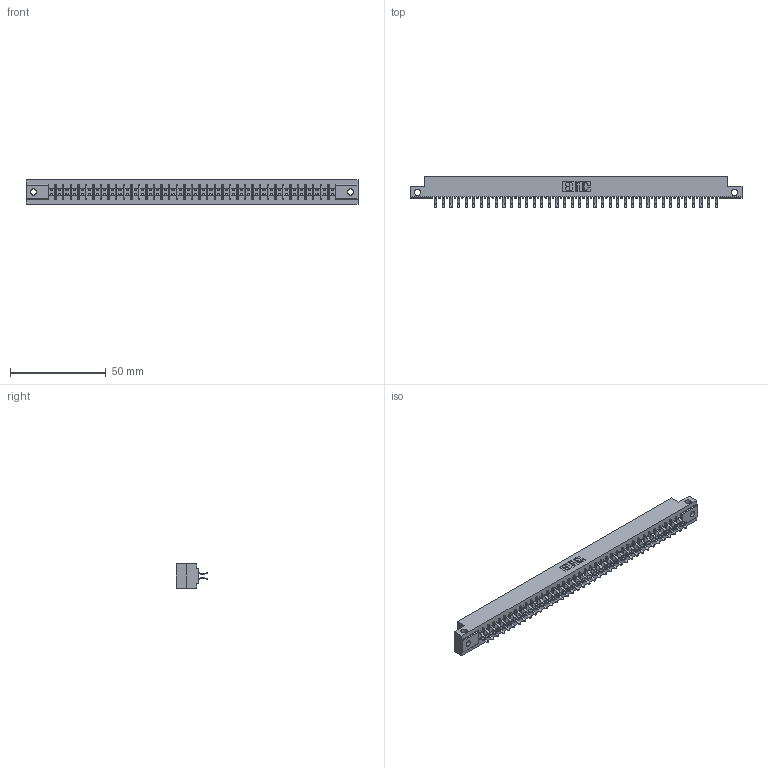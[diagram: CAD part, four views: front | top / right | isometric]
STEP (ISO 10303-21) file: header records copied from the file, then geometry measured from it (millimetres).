
FILE_DESCRIPTION (( 'STEP AP203' ), '1' );
FILE_NAME ('305-076-556-512.STEP', '2020-09-20T00:46:34', ( '' ), ( '' ), 'SwSTEP 2.0', 'SolidWorks 2020', '' );
FILE_SCHEMA (( 'CONFIG_CONTROL_DESIGN' ));
Length unit declared in the file: inch
Products named in the file (3): 305-076-556-512; 305 Part_.128 Dia; 305-290-001_556
Assembly tree (77 placements, depth 2):
  305-076-556-512
    305 Part_.128 Dia
    305-290-001_556  x76
Bounding box: 173.58 x 16.64 x 12.7 mm (x, y, z)
Volume: 17346.4 mm3; surface area: 22923.4 mm2
Topology: 77 solids, 77 shells, 4384 faces, 12626 edges, 8208 vertices
Faces by surface type: plane 2424, cylinder 1808, sphere 152
Entity records: 42259 total; most frequent: CARTESIAN_POINT 7044, ORIENTED_EDGE 6948, DIRECTION 6760, EDGE_CURVE 3474, LINE 2784, VECTOR 2784, VERTEX_POINT 2208, AXIS2_PLACEMENT_3D 1988
